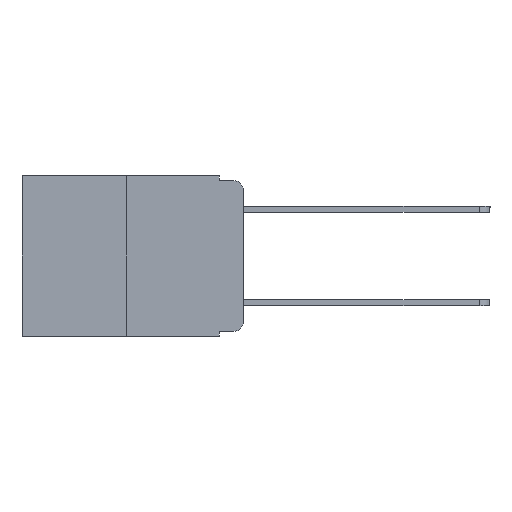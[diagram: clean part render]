
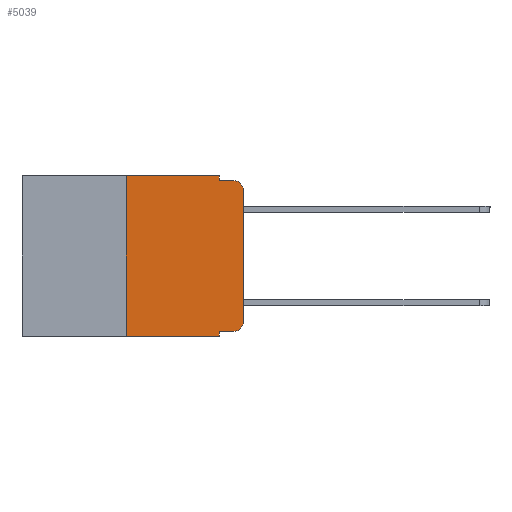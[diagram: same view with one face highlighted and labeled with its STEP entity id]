
A CAD part, left-side view. The second image highlights one B-rep face of the part: STEP entity #5039.
In plain terms, the highlighted planar face has unit normal (-1, 0, 0).
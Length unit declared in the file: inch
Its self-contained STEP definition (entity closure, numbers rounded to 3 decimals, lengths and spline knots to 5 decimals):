
#21 = CARTESIAN_POINT ( 'NONE',  ( 0., 0.051, 0. ) ) ;
#502 = DIRECTION ( 'NONE',  ( 0., 0., 1. ) ) ;
#564 = CARTESIAN_POINT ( 'NONE',  ( 0., 0.051, 0. ) ) ;
#953 = EDGE_CURVE ( 'NONE', #22840, #12799, #4146, .T. ) ;
#1094 = ORIENTED_EDGE ( 'NONE', *, *, #6232, .T. ) ;
#1653 = DIRECTION ( 'NONE',  ( 0., 0., -1. ) ) ;
#2029 = EDGE_LOOP ( 'NONE', ( #1094, #18143, #20454, #11508, #12303, #17902, #17900, #8707, #14006, #10388 ) ) ;
#2388 = CIRCLE ( 'NONE', #9210, 0.02 ) ;
#2608 = LINE ( 'NONE', #564, #17547 ) ;
#2725 = LINE ( 'NONE', #9973, #4995 ) ;
#2820 = CARTESIAN_POINT ( 'NONE',  ( 0., 0., -0.313 ) ) ;
#3237 = EDGE_CURVE ( 'NONE', #11776, #21528, #9811, .T. ) ;
#3447 = DIRECTION ( 'NONE',  ( 0., 0., -1. ) ) ;
#3679 = EDGE_CURVE ( 'NONE', #10585, #10729, #2725, .T. ) ;
#3836 = AXIS2_PLACEMENT_3D ( 'NONE', #13909, #10453, #3447 ) ;
#4146 = LINE ( 'NONE', #9016, #14750 ) ;
#4355 = CARTESIAN_POINT ( 'NONE',  ( 0., 0.02, -0.03 ) ) ;
#4589 = CARTESIAN_POINT ( 'NONE',  ( 0., 0.473, 0. ) ) ;
#4995 = VECTOR ( 'NONE', #16500, 39.37008 ) ;
#5039 = ADVANCED_FACE ( 'NONE', ( #17606 ), #6657, .F. ) ;
#5901 = DIRECTION ( 'NONE',  ( -1., 0., 0. ) ) ;
#5973 = CARTESIAN_POINT ( 'NONE',  ( 0., 0., -0.03 ) ) ;
#6090 = VERTEX_POINT ( 'NONE', #21 ) ;
#6223 = CARTESIAN_POINT ( 'NONE',  ( 0., 0., 0. ) ) ;
#6232 = EDGE_CURVE ( 'NONE', #12340, #10667, #22539, .T. ) ;
#6657 = PLANE ( 'NONE',  #3836 ) ;
#7465 = EDGE_CURVE ( 'NONE', #10585, #22213, #22070, .T. ) ;
#8576 = AXIS2_PLACEMENT_3D ( 'NONE', #4355, #20910, #15075 ) ;
#8707 = ORIENTED_EDGE ( 'NONE', *, *, #21119, .F. ) ;
#9016 = CARTESIAN_POINT ( 'NONE',  ( 0., 0.051, -0.01 ) ) ;
#9210 = AXIS2_PLACEMENT_3D ( 'NONE', #9460, #5901, #1653 ) ;
#9460 = CARTESIAN_POINT ( 'NONE',  ( 0., 0.02, -0.313 ) ) ;
#9639 = LINE ( 'NONE', #20363, #18312 ) ;
#9811 = LINE ( 'NONE', #10047, #17515 ) ;
#9973 = CARTESIAN_POINT ( 'NONE',  ( 0., 0.25, 0. ) ) ;
#10047 = CARTESIAN_POINT ( 'NONE',  ( 0., 0.051, -0.333 ) ) ;
#10388 = ORIENTED_EDGE ( 'NONE', *, *, #21499, .T. ) ;
#10453 = DIRECTION ( 'NONE',  ( 1., 0., 0. ) ) ;
#10585 = VERTEX_POINT ( 'NONE', #16670 ) ;
#10667 = VERTEX_POINT ( 'NONE', #5973 ) ;
#10729 = VERTEX_POINT ( 'NONE', #22753 ) ;
#11508 = ORIENTED_EDGE ( 'NONE', *, *, #20129, .F. ) ;
#11515 = VECTOR ( 'NONE', #16341, 39.37008 ) ;
#11693 = EDGE_CURVE ( 'NONE', #10667, #12799, #19250, .T. ) ;
#11776 = VERTEX_POINT ( 'NONE', #23155 ) ;
#12303 = ORIENTED_EDGE ( 'NONE', *, *, #23480, .F. ) ;
#12340 = VERTEX_POINT ( 'NONE', #2820 ) ;
#12799 = VERTEX_POINT ( 'NONE', #21129 ) ;
#13082 = DIRECTION ( 'NONE',  ( 0., 0., -1. ) ) ;
#13909 = CARTESIAN_POINT ( 'NONE',  ( 0., 0.473, 0. ) ) ;
#14006 = ORIENTED_EDGE ( 'NONE', *, *, #3237, .T. ) ;
#14182 = DIRECTION ( 'NONE',  ( 0., -1., 0. ) ) ;
#14232 = VECTOR ( 'NONE', #14182, 39.37008 ) ;
#14750 = VECTOR ( 'NONE', #21761, 39.37008 ) ;
#15075 = DIRECTION ( 'NONE',  ( 0., 0., -1. ) ) ;
#16038 = VECTOR ( 'NONE', #502, 39.37008 ) ;
#16195 = CARTESIAN_POINT ( 'NONE',  ( 0., 0.051, -0.343 ) ) ;
#16341 = DIRECTION ( 'NONE',  ( 0., -1., 0. ) ) ;
#16500 = DIRECTION ( 'NONE',  ( 0., 0., 1. ) ) ;
#16670 = CARTESIAN_POINT ( 'NONE',  ( 0., 0.25, -0.343 ) ) ;
#16834 = CARTESIAN_POINT ( 'NONE',  ( 0., 0.02, -0.333 ) ) ;
#17308 = DIRECTION ( 'NONE',  ( 0., -1., 0. ) ) ;
#17515 = VECTOR ( 'NONE', #17308, 39.37008 ) ;
#17547 = VECTOR ( 'NONE', #22600, 39.37008 ) ;
#17606 = FACE_OUTER_BOUND ( 'NONE', #2029, .T. ) ;
#17900 = ORIENTED_EDGE ( 'NONE', *, *, #7465, .T. ) ;
#17902 = ORIENTED_EDGE ( 'NONE', *, *, #3679, .F. ) ;
#18143 = ORIENTED_EDGE ( 'NONE', *, *, #11693, .T. ) ;
#18312 = VECTOR ( 'NONE', #13082, 39.37008 ) ;
#19250 = CIRCLE ( 'NONE', #8576, 0.02 ) ;
#20129 = EDGE_CURVE ( 'NONE', #6090, #22840, #2608, .T. ) ;
#20363 = CARTESIAN_POINT ( 'NONE',  ( 0., 0.051, 0. ) ) ;
#20454 = ORIENTED_EDGE ( 'NONE', *, *, #953, .F. ) ;
#20910 = DIRECTION ( 'NONE',  ( -1., 0., 0. ) ) ;
#21119 = EDGE_CURVE ( 'NONE', #11776, #22213, #9639, .T. ) ;
#21129 = CARTESIAN_POINT ( 'NONE',  ( 0., 0.02, -0.01 ) ) ;
#21499 = EDGE_CURVE ( 'NONE', #21528, #12340, #2388, .T. ) ;
#21528 = VERTEX_POINT ( 'NONE', #16834 ) ;
#21761 = DIRECTION ( 'NONE',  ( 0., -1., 0. ) ) ;
#21832 = CARTESIAN_POINT ( 'NONE',  ( 0., 0.473, -0.343 ) ) ;
#22070 = LINE ( 'NONE', #21832, #11515 ) ;
#22213 = VERTEX_POINT ( 'NONE', #16195 ) ;
#22245 = CARTESIAN_POINT ( 'NONE',  ( 0., 0.051, -0.01 ) ) ;
#22539 = LINE ( 'NONE', #6223, #16038 ) ;
#22600 = DIRECTION ( 'NONE',  ( 0., 0., -1. ) ) ;
#22753 = CARTESIAN_POINT ( 'NONE',  ( 0., 0.25, 0. ) ) ;
#22840 = VERTEX_POINT ( 'NONE', #22245 ) ;
#23155 = CARTESIAN_POINT ( 'NONE',  ( 0., 0.051, -0.333 ) ) ;
#23239 = LINE ( 'NONE', #4589, #14232 ) ;
#23480 = EDGE_CURVE ( 'NONE', #10729, #6090, #23239, .T. ) ;
